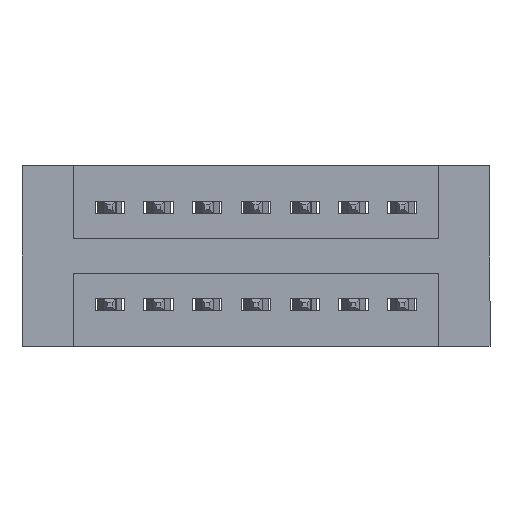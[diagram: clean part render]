
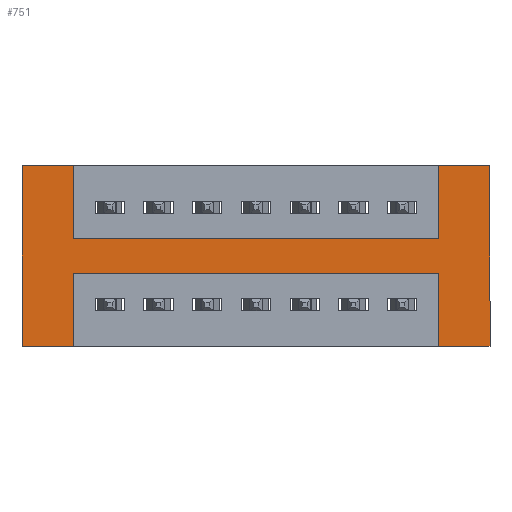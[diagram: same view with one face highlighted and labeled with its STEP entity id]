
A CAD part, front view. The second image highlights one B-rep face of the part: STEP entity #751.
In plain terms, the highlighted planar face has unit normal (0, -1, 0).
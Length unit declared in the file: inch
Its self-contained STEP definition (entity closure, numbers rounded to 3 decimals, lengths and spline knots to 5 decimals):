
#108 = ORIENTED_EDGE ( 'NONE', *, *, #5834, .F. ) ;
#188 = EDGE_CURVE ( 'NONE', #9718, #1835, #3124, .T. ) ;
#208 = CARTESIAN_POINT ( 'NONE',  ( 0.2875, 0., 0. ) ) ;
#215 = CARTESIAN_POINT ( 'NONE',  ( 0.3925, 0., 0. ) ) ;
#270 = VECTOR ( 'NONE', #3155, 39.37008 ) ;
#343 = PLANE ( 'NONE',  #7994 ) ;
#402 = CARTESIAN_POINT ( 'NONE',  ( 0.3925, 0., -0.15 ) ) ;
#437 = EDGE_CURVE ( 'NONE', #8529, #1148, #1019, .T. ) ;
#528 = VECTOR ( 'NONE', #649, 39.37008 ) ;
#632 = VECTOR ( 'NONE', #4832, 39.37008 ) ;
#649 = DIRECTION ( 'NONE',  ( -1., 0., 0. ) ) ;
#751 = ADVANCED_FACE ( 'NONE', ( #3982 ), #343, .T. ) ;
#851 = ORIENTED_EDGE ( 'NONE', *, *, #437, .F. ) ;
#852 = CARTESIAN_POINT ( 'NONE',  ( 1.1425, 0., -0.37 ) ) ;
#1019 = LINE ( 'NONE', #9180, #3762 ) ;
#1148 = VERTEX_POINT ( 'NONE', #2917 ) ;
#1250 = LINE ( 'NONE', #3220, #1725 ) ;
#1364 = LINE ( 'NONE', #208, #632 ) ;
#1422 = ORIENTED_EDGE ( 'NONE', *, *, #9287, .F. ) ;
#1523 = DIRECTION ( 'NONE',  ( -1., 0., 0. ) ) ;
#1567 = EDGE_CURVE ( 'NONE', #1148, #3790, #6858, .T. ) ;
#1679 = LINE ( 'NONE', #5337, #6313 ) ;
#1725 = VECTOR ( 'NONE', #4261, 39.37008 ) ;
#1769 = CARTESIAN_POINT ( 'NONE',  ( 0., 0., 0. ) ) ;
#1802 = LINE ( 'NONE', #1769, #270 ) ;
#1835 = VERTEX_POINT ( 'NONE', #9653 ) ;
#1873 = ORIENTED_EDGE ( 'NONE', *, *, #7202, .F. ) ;
#1878 = CARTESIAN_POINT ( 'NONE',  ( 0.3925, 0., -0.37 ) ) ;
#1956 = CARTESIAN_POINT ( 'NONE',  ( 0.3925, 0., -0.22 ) ) ;
#2037 = CARTESIAN_POINT ( 'NONE',  ( 0., 0., 0. ) ) ;
#2185 = ORIENTED_EDGE ( 'NONE', *, *, #2711, .F. ) ;
#2225 = VERTEX_POINT ( 'NONE', #7306 ) ;
#2455 = ORIENTED_EDGE ( 'NONE', *, *, #9091, .F. ) ;
#2543 = LINE ( 'NONE', #8165, #528 ) ;
#2711 = EDGE_CURVE ( 'NONE', #4095, #3678, #2809, .T. ) ;
#2763 = EDGE_CURVE ( 'NONE', #2225, #3790, #1250, .T. ) ;
#2809 = LINE ( 'NONE', #3196, #9519 ) ;
#2917 = CARTESIAN_POINT ( 'NONE',  ( 1.1425, 0., 0. ) ) ;
#2973 = DIRECTION ( 'NONE',  ( 0., 0., -1. ) ) ;
#3040 = CARTESIAN_POINT ( 'NONE',  ( 0.3925, 0., 0. ) ) ;
#3124 = LINE ( 'NONE', #852, #8006 ) ;
#3155 = DIRECTION ( 'NONE',  ( 1., 0., 0. ) ) ;
#3196 = CARTESIAN_POINT ( 'NONE',  ( 0.3925, 0., -0.37 ) ) ;
#3220 = CARTESIAN_POINT ( 'NONE',  ( 1.2475, 0., 0. ) ) ;
#3371 = EDGE_CURVE ( 'NONE', #1835, #4095, #7350, .T. ) ;
#3384 = CARTESIAN_POINT ( 'NONE',  ( 0., 0., -0.37 ) ) ;
#3426 = VECTOR ( 'NONE', #6665, 39.37008 ) ;
#3678 = VERTEX_POINT ( 'NONE', #1878 ) ;
#3762 = VECTOR ( 'NONE', #7747, 39.37008 ) ;
#3790 = VERTEX_POINT ( 'NONE', #4681 ) ;
#3845 = DIRECTION ( 'NONE',  ( 0., 0., 1. ) ) ;
#3928 = VECTOR ( 'NONE', #5596, 39.37008 ) ;
#3960 = DIRECTION ( 'NONE',  ( 0., 0., -1. ) ) ;
#3982 = FACE_OUTER_BOUND ( 'NONE', #7511, .T. ) ;
#4095 = VERTEX_POINT ( 'NONE', #1956 ) ;
#4142 = ORIENTED_EDGE ( 'NONE', *, *, #3371, .F. ) ;
#4261 = DIRECTION ( 'NONE',  ( 0., 0., 1. ) ) ;
#4681 = CARTESIAN_POINT ( 'NONE',  ( 1.2475, 0., 0. ) ) ;
#4766 = ORIENTED_EDGE ( 'NONE', *, *, #9545, .F. ) ;
#4832 = DIRECTION ( 'NONE',  ( 0., 0., -1. ) ) ;
#5067 = ORIENTED_EDGE ( 'NONE', *, *, #1567, .F. ) ;
#5337 = CARTESIAN_POINT ( 'NONE',  ( 0., 0., -0.37 ) ) ;
#5596 = DIRECTION ( 'NONE',  ( 1., 0., 0. ) ) ;
#5774 = CARTESIAN_POINT ( 'NONE',  ( 0.3925, 0., -0.22 ) ) ;
#5834 = EDGE_CURVE ( 'NONE', #2225, #9718, #2543, .T. ) ;
#5849 = CARTESIAN_POINT ( 'NONE',  ( 1.1425, 0., -0.37 ) ) ;
#5969 = LINE ( 'NONE', #402, #3928 ) ;
#5972 = DIRECTION ( 'NONE',  ( 0., 0., -1. ) ) ;
#6052 = LINE ( 'NONE', #3040, #7948 ) ;
#6313 = VECTOR ( 'NONE', #1523, 39.37008 ) ;
#6462 = EDGE_CURVE ( 'NONE', #8576, #8827, #1364, .T. ) ;
#6570 = ORIENTED_EDGE ( 'NONE', *, *, #188, .F. ) ;
#6665 = DIRECTION ( 'NONE',  ( -1., 0., 0. ) ) ;
#6858 = LINE ( 'NONE', #2037, #9801 ) ;
#7202 = EDGE_CURVE ( 'NONE', #8692, #8529, #5969, .T. ) ;
#7306 = CARTESIAN_POINT ( 'NONE',  ( 1.2475, 0., -0.37 ) ) ;
#7349 = CARTESIAN_POINT ( 'NONE',  ( 1.1425, 0., -0.15 ) ) ;
#7350 = LINE ( 'NONE', #5774, #3426 ) ;
#7497 = ORIENTED_EDGE ( 'NONE', *, *, #6462, .T. ) ;
#7511 = EDGE_LOOP ( 'NONE', ( #8179, #5067, #851, #1873, #4766, #2455, #7497, #1422, #2185, #4142, #6570, #108 ) ) ;
#7531 = DIRECTION ( 'NONE',  ( 1., 0., 0. ) ) ;
#7571 = VERTEX_POINT ( 'NONE', #215 ) ;
#7747 = DIRECTION ( 'NONE',  ( 0., 0., 1. ) ) ;
#7948 = VECTOR ( 'NONE', #2973, 39.37008 ) ;
#7994 = AXIS2_PLACEMENT_3D ( 'NONE', #3384, #8726, #5972 ) ;
#8006 = VECTOR ( 'NONE', #3845, 39.37008 ) ;
#8165 = CARTESIAN_POINT ( 'NONE',  ( 0., 0., -0.37 ) ) ;
#8179 = ORIENTED_EDGE ( 'NONE', *, *, #2763, .T. ) ;
#8529 = VERTEX_POINT ( 'NONE', #7349 ) ;
#8576 = VERTEX_POINT ( 'NONE', #9117 ) ;
#8692 = VERTEX_POINT ( 'NONE', #9737 ) ;
#8726 = DIRECTION ( 'NONE',  ( 0., -1., 0. ) ) ;
#8827 = VERTEX_POINT ( 'NONE', #9781 ) ;
#9091 = EDGE_CURVE ( 'NONE', #8576, #7571, #1802, .T. ) ;
#9117 = CARTESIAN_POINT ( 'NONE',  ( 0.2875, 0., 0. ) ) ;
#9180 = CARTESIAN_POINT ( 'NONE',  ( 1.1425, 0., 0. ) ) ;
#9287 = EDGE_CURVE ( 'NONE', #3678, #8827, #1679, .T. ) ;
#9519 = VECTOR ( 'NONE', #3960, 39.37008 ) ;
#9545 = EDGE_CURVE ( 'NONE', #7571, #8692, #6052, .T. ) ;
#9653 = CARTESIAN_POINT ( 'NONE',  ( 1.1425, 0., -0.22 ) ) ;
#9718 = VERTEX_POINT ( 'NONE', #5849 ) ;
#9737 = CARTESIAN_POINT ( 'NONE',  ( 0.3925, 0., -0.15 ) ) ;
#9781 = CARTESIAN_POINT ( 'NONE',  ( 0.2875, 0., -0.37 ) ) ;
#9801 = VECTOR ( 'NONE', #7531, 39.37008 ) ;
